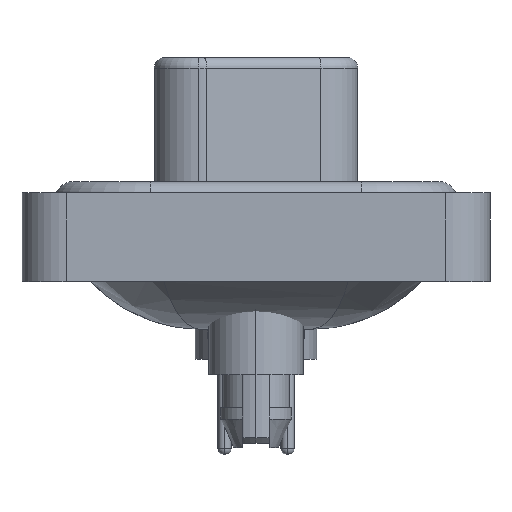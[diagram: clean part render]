
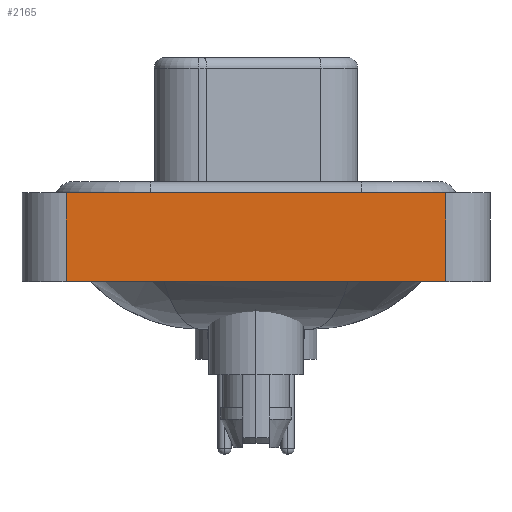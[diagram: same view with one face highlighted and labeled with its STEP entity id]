
A CAD part, left-side view. The second image highlights one B-rep face of the part: STEP entity #2165.
In plain terms, the highlighted planar face has unit normal (-1, 0, 0).
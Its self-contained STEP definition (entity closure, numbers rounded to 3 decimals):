
#337 = ORIENTED_EDGE ( 'NONE', *, *, #6228, .T. ) ;
#437 = AXIS2_PLACEMENT_3D ( 'NONE', #11291, #11095, #4211 ) ;
#448 = CARTESIAN_POINT ( 'NONE',  ( -7.25, -8.55, 0.4 ) ) ;
#612 = CARTESIAN_POINT ( 'NONE',  ( -7.25, 8.55, -3.6 ) ) ;
#1057 = LINE ( 'NONE', #1158, #14976 ) ;
#1158 = CARTESIAN_POINT ( 'NONE',  ( -7.25, -8.55, -3.6 ) ) ;
#1169 = EDGE_CURVE ( 'NONE', #8168, #7533, #13659, .T. ) ;
#1614 = EDGE_CURVE ( 'NONE', #17801, #2252, #5251, .T. ) ;
#2165 = ADVANCED_FACE ( 'NONE', ( #5601 ), #18300, .T. ) ;
#2252 = VERTEX_POINT ( 'NONE', #448 ) ;
#2424 = CARTESIAN_POINT ( 'NONE',  ( -7.25, -8.55, -3.6 ) ) ;
#3539 = ORIENTED_EDGE ( 'NONE', *, *, #1169, .T. ) ;
#4211 = DIRECTION ( 'NONE',  ( 0., 0., 1. ) ) ;
#4884 = VECTOR ( 'NONE', #16656, 1000. ) ;
#5062 = ORIENTED_EDGE ( 'NONE', *, *, #1614, .F. ) ;
#5251 = LINE ( 'NONE', #8143, #18335 ) ;
#5601 = FACE_OUTER_BOUND ( 'NONE', #10103, .T. ) ;
#6228 = EDGE_CURVE ( 'NONE', #7533, #2252, #1057, .T. ) ;
#7323 = CARTESIAN_POINT ( 'NONE',  ( -7.25, 8.55, -3.6 ) ) ;
#7533 = VERTEX_POINT ( 'NONE', #2424 ) ;
#7766 = EDGE_CURVE ( 'NONE', #8168, #17801, #17522, .T. ) ;
#7930 = CARTESIAN_POINT ( 'NONE',  ( -7.25, 8.55, 0.4 ) ) ;
#7954 = DIRECTION ( 'NONE',  ( 0., -1., 0. ) ) ;
#8143 = CARTESIAN_POINT ( 'NONE',  ( -7.25, -8.55, 0.4 ) ) ;
#8168 = VERTEX_POINT ( 'NONE', #7323 ) ;
#9460 = DIRECTION ( 'NONE',  ( 0., 0., 1. ) ) ;
#10103 = EDGE_LOOP ( 'NONE', ( #337, #5062, #10880, #3539 ) ) ;
#10854 = CARTESIAN_POINT ( 'NONE',  ( -7.25, -8.55, -3.6 ) ) ;
#10880 = ORIENTED_EDGE ( 'NONE', *, *, #7766, .F. ) ;
#11095 = DIRECTION ( 'NONE',  ( -1., 0., 0. ) ) ;
#11291 = CARTESIAN_POINT ( 'NONE',  ( -7.25, -8.55, -3.6 ) ) ;
#13659 = LINE ( 'NONE', #10854, #4884 ) ;
#14976 = VECTOR ( 'NONE', #9460, 1000. ) ;
#16284 = DIRECTION ( 'NONE',  ( 0., 0., 1. ) ) ;
#16656 = DIRECTION ( 'NONE',  ( 0., -1., 0. ) ) ;
#17522 = LINE ( 'NONE', #612, #17547 ) ;
#17547 = VECTOR ( 'NONE', #16284, 1000. ) ;
#17801 = VERTEX_POINT ( 'NONE', #7930 ) ;
#18300 = PLANE ( 'NONE',  #437 ) ;
#18335 = VECTOR ( 'NONE', #7954, 1000. ) ;
